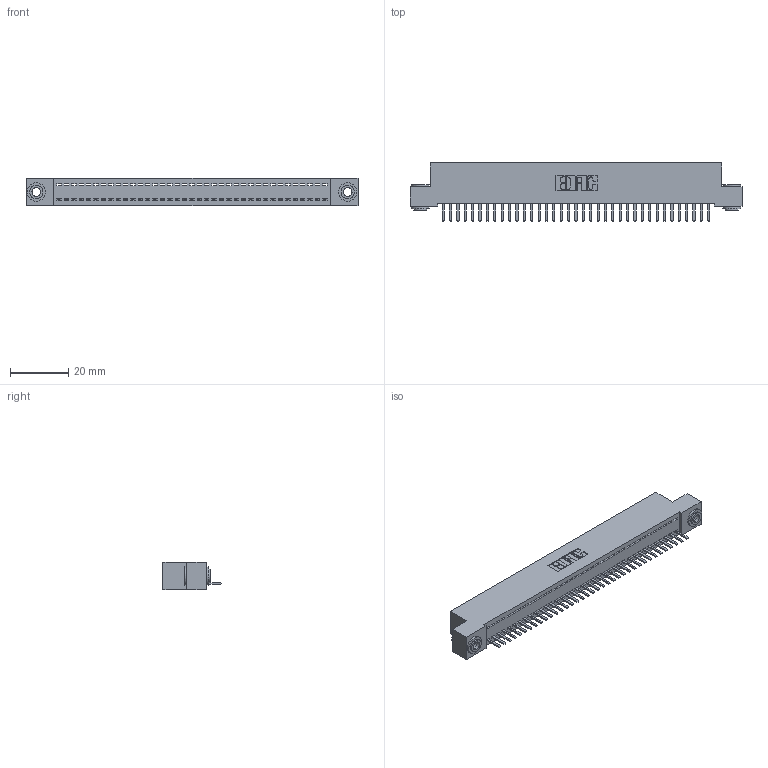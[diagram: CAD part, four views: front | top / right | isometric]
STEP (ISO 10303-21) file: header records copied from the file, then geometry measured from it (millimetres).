
FILE_DESCRIPTION (( 'STEP AP203' ), '1' );
FILE_NAME ('342-037-520-103.STEP', '2018-08-11T21:04:48', ( '' ), ( '' ), 'SwSTEP 2.0', 'SolidWorks 2016', '' );
FILE_SCHEMA (( 'CONFIG_CONTROL_DESIGN' ));
Length unit declared in the file: inch
Products named in the file (4): 342-250-002_345-250-002-102; 342-037-520-103; 342 Part_.156 TH; 345-292-001_345-293-120
Assembly tree (40 placements, depth 2):
  342-037-520-103
    342 Part_.156 TH
    345-292-001_345-293-120  x37
    342-250-002_345-250-002-102  x2
Bounding box: 114.3 x 20.02 x 9.4 mm (x, y, z)
Volume: 9919.8 mm3; surface area: 14359.2 mm2
Topology: 40 solids, 40 shells, 2442 faces, 7183 edges, 4686 vertices
Faces by surface type: plane 1704, cylinder 730, cone 8
Entity records: 23898 total; most frequent: CARTESIAN_POINT 4112, ORIENTED_EDGE 4066, DIRECTION 3501, EDGE_CURVE 2033, VECTOR 1877, LINE 1877, VERTEX_POINT 1350, AXIS2_PLACEMENT_3D 812
